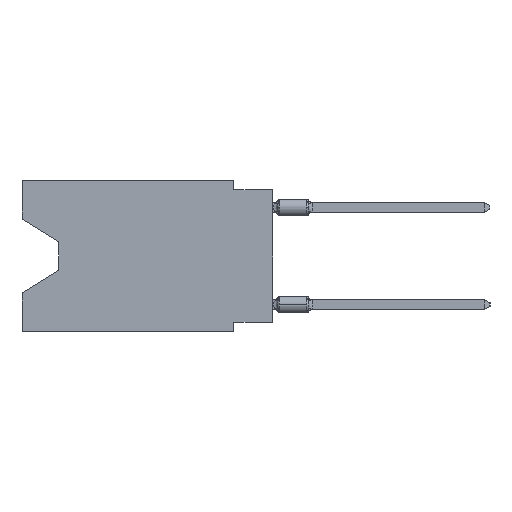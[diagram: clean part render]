
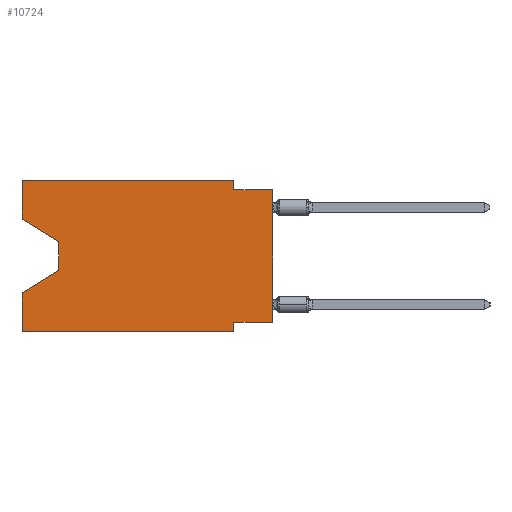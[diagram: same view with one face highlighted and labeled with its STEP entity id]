
A CAD part, left-side view. The second image highlights one B-rep face of the part: STEP entity #10724.
In plain terms, the highlighted planar face has unit normal (-1, 0, 0).
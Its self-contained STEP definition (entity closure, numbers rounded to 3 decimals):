
#1080 = VERTEX_POINT ( 'NONE', #25039 ) ;
#1875 = CARTESIAN_POINT ( 'NONE',  ( 0., 0., 0. ) ) ;
#2643 = CARTESIAN_POINT ( 'NONE',  ( 0., 2.54, -9.906 ) ) ;
#3117 = CARTESIAN_POINT ( 'NONE',  ( 0., 16.383, 0. ) ) ;
#3214 = LINE ( 'NONE', #14796, #6511 ) ;
#3416 = ORIENTED_EDGE ( 'NONE', *, *, #18294, .T. ) ;
#3980 = EDGE_CURVE ( 'NONE', #9440, #7380, #4135, .T. ) ;
#4039 = CARTESIAN_POINT ( 'NONE',  ( 0., 2.54, -9.271 ) ) ;
#4099 = CARTESIAN_POINT ( 'NONE',  ( 0., 16.383, 0. ) ) ;
#4130 = LINE ( 'NONE', #1875, #20507 ) ;
#4135 = LINE ( 'NONE', #13320, #20320 ) ;
#4429 = EDGE_CURVE ( 'NONE', #4454, #11939, #25531, .T. ) ;
#4454 = VERTEX_POINT ( 'NONE', #25375 ) ;
#4691 = DIRECTION ( 'NONE',  ( 0., -1., 0. ) ) ;
#4849 = CARTESIAN_POINT ( 'NONE',  ( 0., 13.97, -4.013 ) ) ;
#5042 = AXIS2_PLACEMENT_3D ( 'NONE', #4099, #12983, #13284 ) ;
#5577 = LINE ( 'NONE', #7992, #10837 ) ;
#5599 = CARTESIAN_POINT ( 'NONE',  ( 0., 16.383, -9.906 ) ) ;
#5784 = EDGE_CURVE ( 'NONE', #13580, #15376, #5577, .T. ) ;
#5995 = CARTESIAN_POINT ( 'NONE',  ( 0., 16.383, -7.36 ) ) ;
#6349 = FACE_OUTER_BOUND ( 'NONE', #8254, .T. ) ;
#6511 = VECTOR ( 'NONE', #22053, 1000. ) ;
#6652 = LINE ( 'NONE', #15857, #8504 ) ;
#7090 = DIRECTION ( 'NONE',  ( 0., -1., 0. ) ) ;
#7380 = VERTEX_POINT ( 'NONE', #24955 ) ;
#7456 = CARTESIAN_POINT ( 'NONE',  ( 0., 13.97, -5.893 ) ) ;
#7654 = EDGE_CURVE ( 'NONE', #7380, #1080, #3214, .T. ) ;
#7674 = VERTEX_POINT ( 'NONE', #5599 ) ;
#7850 = VERTEX_POINT ( 'NONE', #19927 ) ;
#7957 = EDGE_CURVE ( 'NONE', #24023, #4454, #14179, .T. ) ;
#7977 = VECTOR ( 'NONE', #11921, 1000. ) ;
#7992 = CARTESIAN_POINT ( 'NONE',  ( 0., 0., -9.271 ) ) ;
#8254 = EDGE_LOOP ( 'NONE', ( #10817, #18455, #10824, #27066, #27169, #22007, #21308, #3416, #28340, #29278, #29072, #27037 ) ) ;
#8504 = VECTOR ( 'NONE', #4691, 1000. ) ;
#8917 = EDGE_CURVE ( 'NONE', #7674, #9461, #16661, .T. ) ;
#8934 = CARTESIAN_POINT ( 'NONE',  ( 0., 16.383, -2.546 ) ) ;
#9440 = VERTEX_POINT ( 'NONE', #22766 ) ;
#9461 = VERTEX_POINT ( 'NONE', #5995 ) ;
#9599 = DIRECTION ( 'NONE',  ( 0., 0., 1. ) ) ;
#9655 = CARTESIAN_POINT ( 'NONE',  ( 0., 16.383, -2.546 ) ) ;
#9867 = CARTESIAN_POINT ( 'NONE',  ( 0., 16.383, 0. ) ) ;
#10212 = VECTOR ( 'NONE', #23264, 1000. ) ;
#10724 = ADVANCED_FACE ( 'NONE', ( #6349 ), #15550, .F. ) ;
#10817 = ORIENTED_EDGE ( 'NONE', *, *, #7957, .T. ) ;
#10824 = ORIENTED_EDGE ( 'NONE', *, *, #27648, .T. ) ;
#10837 = VECTOR ( 'NONE', #21595, 1000. ) ;
#11921 = DIRECTION ( 'NONE',  ( 0., -0.855, -0.519 ) ) ;
#11939 = VERTEX_POINT ( 'NONE', #15412 ) ;
#11959 = VECTOR ( 'NONE', #16498, 1000. ) ;
#12451 = VERTEX_POINT ( 'NONE', #18362 ) ;
#12902 = VECTOR ( 'NONE', #16648, 1000. ) ;
#12983 = DIRECTION ( 'NONE',  ( 1., 0., 0. ) ) ;
#13284 = DIRECTION ( 'NONE',  ( 0., 0., -1. ) ) ;
#13320 = CARTESIAN_POINT ( 'NONE',  ( 0., 16.383, 0. ) ) ;
#13580 = VERTEX_POINT ( 'NONE', #17798 ) ;
#14179 = LINE ( 'NONE', #9655, #7977 ) ;
#14796 = CARTESIAN_POINT ( 'NONE',  ( 0., 2.54, 0. ) ) ;
#15235 = VECTOR ( 'NONE', #19086, 1000. ) ;
#15311 = VECTOR ( 'NONE', #7090, 1000. ) ;
#15376 = VERTEX_POINT ( 'NONE', #4039 ) ;
#15412 = CARTESIAN_POINT ( 'NONE',  ( 0., 13.97, -5.893 ) ) ;
#15550 = PLANE ( 'NONE',  #5042 ) ;
#15857 = CARTESIAN_POINT ( 'NONE',  ( 0., 16.383, -9.906 ) ) ;
#16498 = DIRECTION ( 'NONE',  ( 0., 0., -1. ) ) ;
#16526 = LINE ( 'NONE', #3117, #17682 ) ;
#16648 = DIRECTION ( 'NONE',  ( 0., 0.855, -0.519 ) ) ;
#16661 = LINE ( 'NONE', #9867, #15235 ) ;
#17682 = VECTOR ( 'NONE', #9599, 1000. ) ;
#17798 = CARTESIAN_POINT ( 'NONE',  ( 0., 0., -9.271 ) ) ;
#18294 = EDGE_CURVE ( 'NONE', #13580, #12451, #4130, .T. ) ;
#18362 = CARTESIAN_POINT ( 'NONE',  ( 0., 0., -0.635 ) ) ;
#18455 = ORIENTED_EDGE ( 'NONE', *, *, #4429, .T. ) ;
#18921 = LINE ( 'NONE', #7456, #12902 ) ;
#19086 = DIRECTION ( 'NONE',  ( 0., 0., 1. ) ) ;
#19467 = EDGE_CURVE ( 'NONE', #7674, #7850, #6652, .T. ) ;
#19518 = DIRECTION ( 'NONE',  ( 0., 0., 1. ) ) ;
#19927 = CARTESIAN_POINT ( 'NONE',  ( 0., 2.54, -9.906 ) ) ;
#20320 = VECTOR ( 'NONE', #27220, 1000. ) ;
#20507 = VECTOR ( 'NONE', #19518, 1000. ) ;
#21308 = ORIENTED_EDGE ( 'NONE', *, *, #5784, .F. ) ;
#21595 = DIRECTION ( 'NONE',  ( 0., 1., 0. ) ) ;
#22007 = ORIENTED_EDGE ( 'NONE', *, *, #27629, .F. ) ;
#22053 = DIRECTION ( 'NONE',  ( 0., 0., -1. ) ) ;
#22766 = CARTESIAN_POINT ( 'NONE',  ( 0., 16.383, 0. ) ) ;
#23097 = LINE ( 'NONE', #27772, #15311 ) ;
#23264 = DIRECTION ( 'NONE',  ( 0., 0., -1. ) ) ;
#24023 = VERTEX_POINT ( 'NONE', #8934 ) ;
#24955 = CARTESIAN_POINT ( 'NONE',  ( 0., 2.54, 0. ) ) ;
#25006 = EDGE_CURVE ( 'NONE', #24023, #9440, #16526, .T. ) ;
#25039 = CARTESIAN_POINT ( 'NONE',  ( 0., 2.54, -0.635 ) ) ;
#25375 = CARTESIAN_POINT ( 'NONE',  ( 0., 13.97, -4.013 ) ) ;
#25531 = LINE ( 'NONE', #4849, #10212 ) ;
#27037 = ORIENTED_EDGE ( 'NONE', *, *, #25006, .F. ) ;
#27066 = ORIENTED_EDGE ( 'NONE', *, *, #8917, .F. ) ;
#27169 = ORIENTED_EDGE ( 'NONE', *, *, #19467, .T. ) ;
#27220 = DIRECTION ( 'NONE',  ( 0., -1., 0. ) ) ;
#27296 = EDGE_CURVE ( 'NONE', #1080, #12451, #23097, .T. ) ;
#27629 = EDGE_CURVE ( 'NONE', #15376, #7850, #28126, .T. ) ;
#27648 = EDGE_CURVE ( 'NONE', #11939, #9461, #18921, .T. ) ;
#27772 = CARTESIAN_POINT ( 'NONE',  ( 0., 0., -0.635 ) ) ;
#28126 = LINE ( 'NONE', #2643, #11959 ) ;
#28340 = ORIENTED_EDGE ( 'NONE', *, *, #27296, .F. ) ;
#29072 = ORIENTED_EDGE ( 'NONE', *, *, #3980, .F. ) ;
#29278 = ORIENTED_EDGE ( 'NONE', *, *, #7654, .F. ) ;
